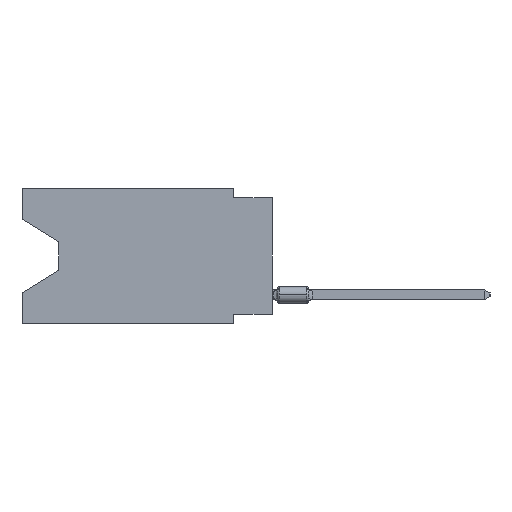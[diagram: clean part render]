
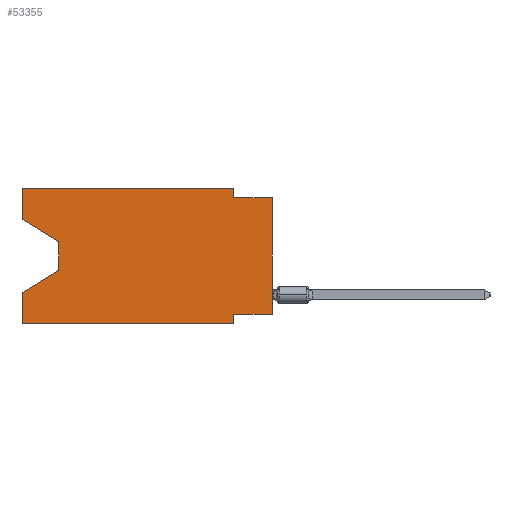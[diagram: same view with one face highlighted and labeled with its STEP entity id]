
A CAD part, left-side view. The second image highlights one B-rep face of the part: STEP entity #53355.
In plain terms, the highlighted planar face has unit normal (-1, 0, 0).
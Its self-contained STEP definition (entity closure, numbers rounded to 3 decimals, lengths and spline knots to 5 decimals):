
#253 = DIRECTION ( 'NONE',  ( 0., -1., 0. ) ) ;
#594 = DIRECTION ( 'NONE',  ( 0., 0., -1. ) ) ;
#934 = VERTEX_POINT ( 'NONE', #20555 ) ;
#986 = EDGE_CURVE ( 'NONE', #3548, #65811, #9016, .T. ) ;
#3082 = ORIENTED_EDGE ( 'NONE', *, *, #41101, .F. ) ;
#3381 = ORIENTED_EDGE ( 'NONE', *, *, #65298, .T. ) ;
#3548 = VERTEX_POINT ( 'NONE', #60913 ) ;
#4157 = CARTESIAN_POINT ( 'NONE',  ( 0., 0.1, 0. ) ) ;
#5883 = CARTESIAN_POINT ( 'NONE',  ( 0., 0.1, -0.35 ) ) ;
#7216 = VECTOR ( 'NONE', #41224, 39.37008 ) ;
#7422 = VERTEX_POINT ( 'NONE', #30902 ) ;
#8600 = DIRECTION ( 'NONE',  ( 0., -1., 0. ) ) ;
#8891 = CARTESIAN_POINT ( 'NONE',  ( 0., 0.645, 0. ) ) ;
#9016 = LINE ( 'NONE', #19186, #7216 ) ;
#9199 = ORIENTED_EDGE ( 'NONE', *, *, #53541, .T. ) ;
#11619 = VECTOR ( 'NONE', #61071, 39.37008 ) ;
#13142 = VERTEX_POINT ( 'NONE', #22409 ) ;
#13196 = CARTESIAN_POINT ( 'NONE',  ( 0., 0.55, -0.212 ) ) ;
#13361 = VERTEX_POINT ( 'NONE', #14322 ) ;
#14322 = CARTESIAN_POINT ( 'NONE',  ( 0., 0.645, -0.35 ) ) ;
#14853 = LINE ( 'NONE', #63781, #27601 ) ;
#14919 = LINE ( 'NONE', #20183, #43104 ) ;
#16722 = CARTESIAN_POINT ( 'NONE',  ( 0., 0.645, 0. ) ) ;
#17090 = LINE ( 'NONE', #5883, #45249 ) ;
#17671 = VECTOR ( 'NONE', #253, 39.37008 ) ;
#18759 = ORIENTED_EDGE ( 'NONE', *, *, #60369, .T. ) ;
#18831 = CARTESIAN_POINT ( 'NONE',  ( 0., 0.645, -0.08025 ) ) ;
#19186 = CARTESIAN_POINT ( 'NONE',  ( 0., 0.55, -0.138 ) ) ;
#19358 = ORIENTED_EDGE ( 'NONE', *, *, #42602, .T. ) ;
#20183 = CARTESIAN_POINT ( 'NONE',  ( 0., 0.645, 0. ) ) ;
#20555 = CARTESIAN_POINT ( 'NONE',  ( 0., 0.1, -0.325 ) ) ;
#20886 = AXIS2_PLACEMENT_3D ( 'NONE', #68566, #48914, #594 ) ;
#21975 = PLANE ( 'NONE',  #20886 ) ;
#22409 = CARTESIAN_POINT ( 'NONE',  ( 0., 0., -0.025 ) ) ;
#23068 = ORIENTED_EDGE ( 'NONE', *, *, #41010, .F. ) ;
#23182 = VECTOR ( 'NONE', #45741, 39.37008 ) ;
#23728 = VECTOR ( 'NONE', #8600, 39.37008 ) ;
#24908 = ORIENTED_EDGE ( 'NONE', *, *, #62546, .F. ) ;
#24921 = VECTOR ( 'NONE', #59254, 39.37008 ) ;
#26411 = VECTOR ( 'NONE', #62912, 39.37008 ) ;
#26899 = DIRECTION ( 'NONE',  ( 0., 0., -1. ) ) ;
#26977 = EDGE_CURVE ( 'NONE', #49055, #13142, #62099, .T. ) ;
#27601 = VECTOR ( 'NONE', #56871, 39.37008 ) ;
#30516 = CARTESIAN_POINT ( 'NONE',  ( 0., 0., -0.325 ) ) ;
#30902 = CARTESIAN_POINT ( 'NONE',  ( 0., 0.645, -0.08025 ) ) ;
#31188 = EDGE_CURVE ( 'NONE', #57028, #934, #63443, .T. ) ;
#33291 = EDGE_CURVE ( 'NONE', #934, #52177, #17090, .T. ) ;
#34846 = CARTESIAN_POINT ( 'NONE',  ( 0., 0., -0.025 ) ) ;
#35607 = DIRECTION ( 'NONE',  ( 0., -0.855, -0.519 ) ) ;
#36464 = ORIENTED_EDGE ( 'NONE', *, *, #31188, .F. ) ;
#36602 = DIRECTION ( 'NONE',  ( 0., 0., 1. ) ) ;
#36624 = ORIENTED_EDGE ( 'NONE', *, *, #64579, .F. ) ;
#41010 = EDGE_CURVE ( 'NONE', #56927, #49055, #46164, .T. ) ;
#41101 = EDGE_CURVE ( 'NONE', #41784, #56927, #48567, .T. ) ;
#41224 = DIRECTION ( 'NONE',  ( 0., 0., -1. ) ) ;
#41251 = ORIENTED_EDGE ( 'NONE', *, *, #986, .T. ) ;
#41447 = ORIENTED_EDGE ( 'NONE', *, *, #26977, .F. ) ;
#41487 = CARTESIAN_POINT ( 'NONE',  ( 0., 0.1, -0.025 ) ) ;
#41622 = LINE ( 'NONE', #53168, #26411 ) ;
#41784 = VERTEX_POINT ( 'NONE', #8891 ) ;
#42393 = VECTOR ( 'NONE', #35607, 39.37008 ) ;
#42602 = EDGE_CURVE ( 'NONE', #7422, #3548, #50653, .T. ) ;
#43104 = VECTOR ( 'NONE', #36602, 39.37008 ) ;
#45249 = VECTOR ( 'NONE', #26899, 39.37008 ) ;
#45619 = CARTESIAN_POINT ( 'NONE',  ( 0., 0.1, 0. ) ) ;
#45741 = DIRECTION ( 'NONE',  ( 0., 0.855, -0.519 ) ) ;
#46056 = ORIENTED_EDGE ( 'NONE', *, *, #33291, .F. ) ;
#46164 = LINE ( 'NONE', #4157, #60057 ) ;
#46981 = CARTESIAN_POINT ( 'NONE',  ( 0., 0.55, -0.212 ) ) ;
#48567 = LINE ( 'NONE', #16722, #17671 ) ;
#48914 = DIRECTION ( 'NONE',  ( 1., 0., 0. ) ) ;
#49055 = VERTEX_POINT ( 'NONE', #41487 ) ;
#49180 = VERTEX_POINT ( 'NONE', #54036 ) ;
#50653 = LINE ( 'NONE', #18831, #42393 ) ;
#51979 = LINE ( 'NONE', #56542, #11619 ) ;
#52177 = VERTEX_POINT ( 'NONE', #66894 ) ;
#53168 = CARTESIAN_POINT ( 'NONE',  ( 0., 0.645, 0. ) ) ;
#53355 = ADVANCED_FACE ( 'NONE', ( #68229 ), #21975, .F. ) ;
#53541 = EDGE_CURVE ( 'NONE', #65811, #49180, #61105, .T. ) ;
#54036 = CARTESIAN_POINT ( 'NONE',  ( 0., 0.645, -0.26975 ) ) ;
#54324 = EDGE_LOOP ( 'NONE', ( #19358, #41251, #9199, #36624, #18759, #46056, #36464, #3381, #41447, #23068, #3082, #24908 ) ) ;
#56542 = CARTESIAN_POINT ( 'NONE',  ( 0., 0.645, -0.35 ) ) ;
#56871 = DIRECTION ( 'NONE',  ( 0., 0., 1. ) ) ;
#56927 = VERTEX_POINT ( 'NONE', #45619 ) ;
#57028 = VERTEX_POINT ( 'NONE', #30516 ) ;
#57894 = CARTESIAN_POINT ( 'NONE',  ( 0., 0., -0.325 ) ) ;
#59254 = DIRECTION ( 'NONE',  ( 0., 1., 0. ) ) ;
#60057 = VECTOR ( 'NONE', #67475, 39.37008 ) ;
#60369 = EDGE_CURVE ( 'NONE', #13361, #52177, #51979, .T. ) ;
#60913 = CARTESIAN_POINT ( 'NONE',  ( 0., 0.55, -0.138 ) ) ;
#61071 = DIRECTION ( 'NONE',  ( 0., -1., 0. ) ) ;
#61105 = LINE ( 'NONE', #13196, #23182 ) ;
#62099 = LINE ( 'NONE', #34846, #23728 ) ;
#62546 = EDGE_CURVE ( 'NONE', #7422, #41784, #14919, .T. ) ;
#62912 = DIRECTION ( 'NONE',  ( 0., 0., 1. ) ) ;
#63443 = LINE ( 'NONE', #57894, #24921 ) ;
#63781 = CARTESIAN_POINT ( 'NONE',  ( 0., 0., 0. ) ) ;
#64579 = EDGE_CURVE ( 'NONE', #13361, #49180, #41622, .T. ) ;
#65298 = EDGE_CURVE ( 'NONE', #57028, #13142, #14853, .T. ) ;
#65811 = VERTEX_POINT ( 'NONE', #46981 ) ;
#66894 = CARTESIAN_POINT ( 'NONE',  ( 0., 0.1, -0.35 ) ) ;
#67475 = DIRECTION ( 'NONE',  ( 0., 0., -1. ) ) ;
#68229 = FACE_OUTER_BOUND ( 'NONE', #54324, .T. ) ;
#68566 = CARTESIAN_POINT ( 'NONE',  ( 0., 0.645, 0. ) ) ;
